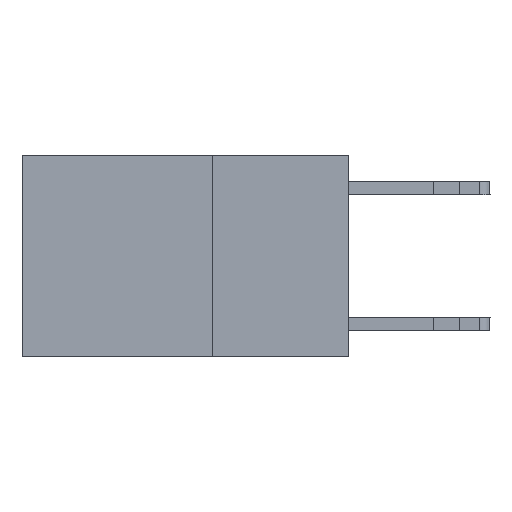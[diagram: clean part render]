
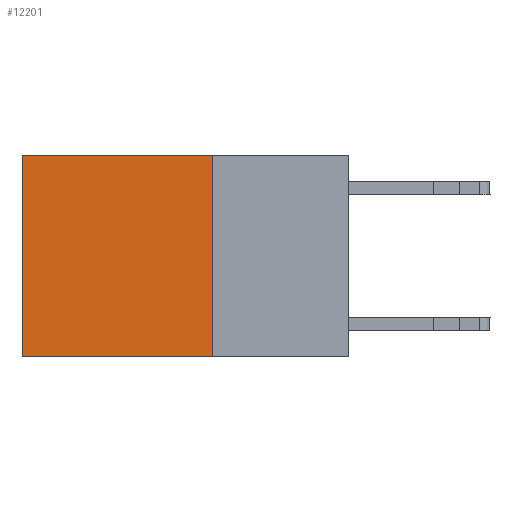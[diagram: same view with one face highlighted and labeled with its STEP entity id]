
A CAD part, left-side view. The second image highlights one B-rep face of the part: STEP entity #12201.
In plain terms, the highlighted planar face has unit normal (-1, 0, 0).
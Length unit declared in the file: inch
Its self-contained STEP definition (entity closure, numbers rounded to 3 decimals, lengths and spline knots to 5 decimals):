
#1073 = CARTESIAN_POINT ( 'NONE',  ( 0.2625, 0.25, 0. ) ) ;
#1135 = VECTOR ( 'NONE', #10795, 39.37008 ) ;
#1236 = CARTESIAN_POINT ( 'NONE',  ( 0.2625, 0.6, -0.37 ) ) ;
#1627 = VERTEX_POINT ( 'NONE', #1236 ) ;
#1682 = EDGE_CURVE ( 'NONE', #7393, #1627, #12027, .T. ) ;
#2104 = DIRECTION ( 'NONE',  ( 0., 1., 0. ) ) ;
#3383 = CARTESIAN_POINT ( 'NONE',  ( 0.2625, 0.6, 0. ) ) ;
#4094 = LINE ( 'NONE', #10201, #6221 ) ;
#4167 = CARTESIAN_POINT ( 'NONE',  ( 0.2625, 0.6, 0. ) ) ;
#4172 = EDGE_LOOP ( 'NONE', ( #11429, #9758, #11242, #6036 ) ) ;
#4499 = EDGE_CURVE ( 'NONE', #8528, #7074, #4094, .T. ) ;
#6036 = ORIENTED_EDGE ( 'NONE', *, *, #4499, .T. ) ;
#6221 = VECTOR ( 'NONE', #2104, 39.37008 ) ;
#6345 = CARTESIAN_POINT ( 'NONE',  ( 0.2625, 0.25, 0. ) ) ;
#7074 = VERTEX_POINT ( 'NONE', #3383 ) ;
#7336 = CARTESIAN_POINT ( 'NONE',  ( 0.2625, 0.25, -0.37 ) ) ;
#7393 = VERTEX_POINT ( 'NONE', #7336 ) ;
#7700 = FACE_OUTER_BOUND ( 'NONE', #4172, .T. ) ;
#7952 = CARTESIAN_POINT ( 'NONE',  ( 0.2625, 0.25, 0. ) ) ;
#8100 = LINE ( 'NONE', #4167, #10686 ) ;
#8136 = LINE ( 'NONE', #1073, #9923 ) ;
#8528 = VERTEX_POINT ( 'NONE', #6345 ) ;
#9655 = CARTESIAN_POINT ( 'NONE',  ( 0.2625, 0.25, -0.37 ) ) ;
#9758 = ORIENTED_EDGE ( 'NONE', *, *, #1682, .F. ) ;
#9923 = VECTOR ( 'NONE', #15437, 39.37008 ) ;
#10201 = CARTESIAN_POINT ( 'NONE',  ( 0.2625, 0.25, 0. ) ) ;
#10433 = DIRECTION ( 'NONE',  ( 1., 0., 0. ) ) ;
#10686 = VECTOR ( 'NONE', #13993, 39.37008 ) ;
#10795 = DIRECTION ( 'NONE',  ( 0., 1., 0. ) ) ;
#11242 = ORIENTED_EDGE ( 'NONE', *, *, #15858, .F. ) ;
#11429 = ORIENTED_EDGE ( 'NONE', *, *, #13989, .T. ) ;
#12027 = LINE ( 'NONE', #9655, #1135 ) ;
#12201 = ADVANCED_FACE ( 'NONE', ( #7700 ), #15104, .F. ) ;
#13063 = AXIS2_PLACEMENT_3D ( 'NONE', #7952, #10433, #15259 ) ;
#13989 = EDGE_CURVE ( 'NONE', #7074, #1627, #8100, .T. ) ;
#13993 = DIRECTION ( 'NONE',  ( 0., 0., -1. ) ) ;
#15104 = PLANE ( 'NONE',  #13063 ) ;
#15259 = DIRECTION ( 'NONE',  ( 0., 0., -1. ) ) ;
#15437 = DIRECTION ( 'NONE',  ( 0., 0., -1. ) ) ;
#15858 = EDGE_CURVE ( 'NONE', #8528, #7393, #8136, .T. ) ;
